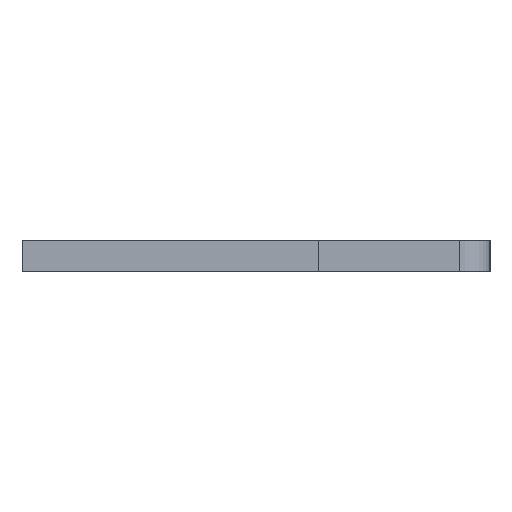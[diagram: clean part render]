
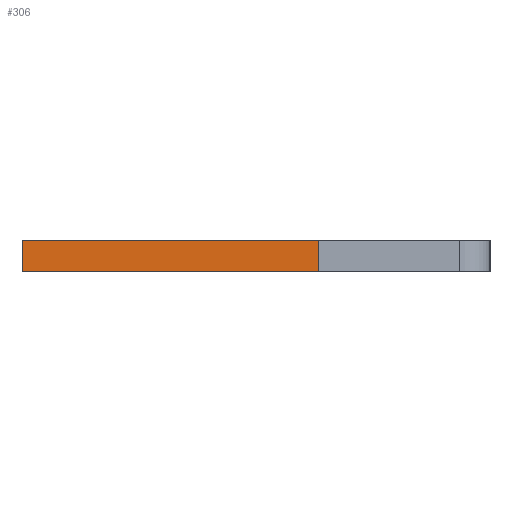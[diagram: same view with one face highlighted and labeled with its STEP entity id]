
A CAD part, left-side view. The second image highlights one B-rep face of the part: STEP entity #306.
In plain terms, the highlighted face is planar.
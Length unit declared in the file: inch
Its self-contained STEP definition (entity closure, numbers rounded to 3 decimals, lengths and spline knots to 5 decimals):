
#47 = DIRECTION ( 'NONE',  ( 1., 0., 0. ) ) ;
#83 = CARTESIAN_POINT ( 'NONE',  ( 0.01, 0.15, -0.04 ) ) ;
#122 = VECTOR ( 'NONE', #929, 39.37008 ) ;
#151 = VECTOR ( 'NONE', #1172, 39.37008 ) ;
#194 = FACE_OUTER_BOUND ( 'NONE', #588, .T. ) ;
#306 = ADVANCED_FACE ( 'NONE', ( #194 ), #540, .F. ) ;
#314 = VERTEX_POINT ( 'NONE', #404 ) ;
#328 = CARTESIAN_POINT ( 'NONE',  ( 0.01, 0.15, -0.04 ) ) ;
#331 = AXIS2_PLACEMENT_3D ( 'NONE', #784, #1255, #47 ) ;
#368 = ORIENTED_EDGE ( 'NONE', *, *, #471, .T. ) ;
#404 = CARTESIAN_POINT ( 'NONE',  ( -0.01, 0.15, -0.04 ) ) ;
#443 = VECTOR ( 'NONE', #1286, 39.37008 ) ;
#471 = EDGE_CURVE ( 'NONE', #1499, #314, #1252, .T. ) ;
#540 = PLANE ( 'NONE',  #331 ) ;
#562 = VERTEX_POINT ( 'NONE', #83 ) ;
#588 = EDGE_LOOP ( 'NONE', ( #368, #964, #1436, #1263 ) ) ;
#601 = EDGE_CURVE ( 'NONE', #1155, #1499, #1413, .T. ) ;
#725 = CARTESIAN_POINT ( 'NONE',  ( 0.01, -0.04, -0.04 ) ) ;
#784 = CARTESIAN_POINT ( 'NONE',  ( 0.01, 0.15, -0.04 ) ) ;
#790 = VECTOR ( 'NONE', #1203, 39.37008 ) ;
#929 = DIRECTION ( 'NONE',  ( 0., 1., 0. ) ) ;
#964 = ORIENTED_EDGE ( 'NONE', *, *, #1075, .F. ) ;
#1037 = CARTESIAN_POINT ( 'NONE',  ( -0.01, 0.15, -0.04 ) ) ;
#1044 = EDGE_CURVE ( 'NONE', #1155, #562, #1351, .T. ) ;
#1058 = CARTESIAN_POINT ( 'NONE',  ( 0.01, -0.04, -0.04 ) ) ;
#1075 = EDGE_CURVE ( 'NONE', #562, #314, #1467, .T. ) ;
#1155 = VERTEX_POINT ( 'NONE', #725 ) ;
#1172 = DIRECTION ( 'NONE',  ( -1., 0., 0. ) ) ;
#1203 = DIRECTION ( 'NONE',  ( -1., 0., 0. ) ) ;
#1252 = LINE ( 'NONE', #1037, #122 ) ;
#1255 = DIRECTION ( 'NONE',  ( 0., 0., 1. ) ) ;
#1263 = ORIENTED_EDGE ( 'NONE', *, *, #601, .T. ) ;
#1286 = DIRECTION ( 'NONE',  ( 0., 1., 0. ) ) ;
#1351 = LINE ( 'NONE', #328, #443 ) ;
#1413 = LINE ( 'NONE', #1058, #151 ) ;
#1431 = CARTESIAN_POINT ( 'NONE',  ( 0.01, 0.15, -0.04 ) ) ;
#1436 = ORIENTED_EDGE ( 'NONE', *, *, #1044, .F. ) ;
#1467 = LINE ( 'NONE', #1431, #790 ) ;
#1468 = CARTESIAN_POINT ( 'NONE',  ( -0.01, -0.04, -0.04 ) ) ;
#1499 = VERTEX_POINT ( 'NONE', #1468 ) ;
